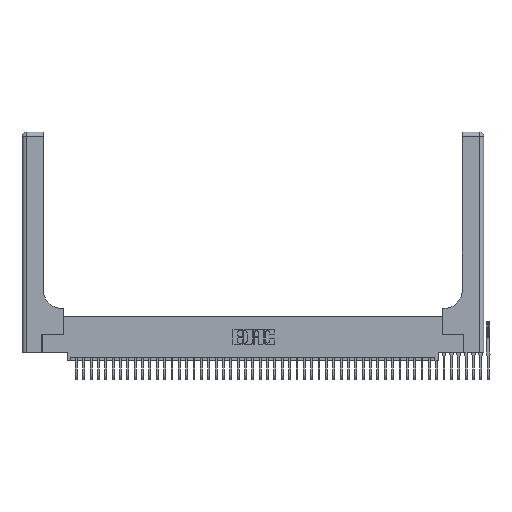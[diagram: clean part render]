
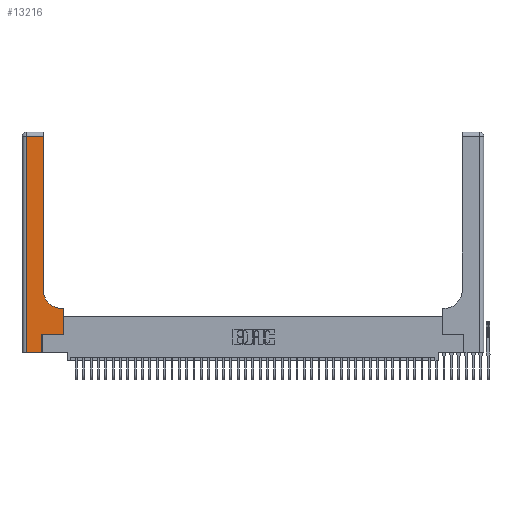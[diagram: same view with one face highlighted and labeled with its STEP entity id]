
A CAD part, top view. The second image highlights one B-rep face of the part: STEP entity #13216.
In plain terms, the highlighted planar face has unit normal (0, 0, 1).
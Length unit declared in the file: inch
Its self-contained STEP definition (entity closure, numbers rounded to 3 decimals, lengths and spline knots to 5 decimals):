
#249 = VECTOR ( 'NONE', #3929, 39.37008 ) ;
#1131 = LINE ( 'NONE', #40847, #33345 ) ;
#1214 = EDGE_CURVE ( 'NONE', #23327, #37470, #10879, .T. ) ;
#1344 = EDGE_CURVE ( 'NONE', #18120, #19431, #21872, .T. ) ;
#1423 = DIRECTION ( 'NONE',  ( -1., 0., 0. ) ) ;
#1444 = VERTEX_POINT ( 'NONE', #2225 ) ;
#2225 = CARTESIAN_POINT ( 'NONE',  ( 0.2915, 2.94, 0.37 ) ) ;
#2936 = LINE ( 'NONE', #36733, #35047 ) ;
#3026 = CARTESIAN_POINT ( 'NONE',  ( 0., 2.94, 0.37 ) ) ;
#3512 = ORIENTED_EDGE ( 'NONE', *, *, #27637, .T. ) ;
#3929 = DIRECTION ( 'NONE',  ( 0., 1., 0. ) ) ;
#4233 = CARTESIAN_POINT ( 'NONE',  ( 0.5415, 0.6, 0.37 ) ) ;
#4406 = DIRECTION ( 'NONE',  ( 0., 0., -1. ) ) ;
#5107 = DIRECTION ( 'NONE',  ( 1., 0., 0. ) ) ;
#5789 = ORIENTED_EDGE ( 'NONE', *, *, #1214, .T. ) ;
#6379 = EDGE_CURVE ( 'NONE', #37470, #1444, #25581, .T. ) ;
#8117 = DIRECTION ( 'NONE',  ( -1., 0., 0. ) ) ;
#8252 = CARTESIAN_POINT ( 'NONE',  ( 0.269, 0.25, 0.37 ) ) ;
#8595 = ORIENTED_EDGE ( 'NONE', *, *, #38573, .T. ) ;
#8697 = EDGE_CURVE ( 'NONE', #21396, #18120, #1131, .T. ) ;
#9582 = DIRECTION ( 'NONE',  ( -1., 0., 0. ) ) ;
#10017 = EDGE_CURVE ( 'NONE', #1444, #25711, #21211, .T. ) ;
#10879 = CIRCLE ( 'NONE', #30761, 0.25 ) ;
#11044 = LINE ( 'NONE', #13742, #19515 ) ;
#12001 = CARTESIAN_POINT ( 'NONE',  ( 0.269, 0.25, 0.37 ) ) ;
#12056 = ORIENTED_EDGE ( 'NONE', *, *, #1344, .T. ) ;
#12397 = LINE ( 'NONE', #12884, #36832 ) ;
#12884 = CARTESIAN_POINT ( 'NONE',  ( 0.06, 3., 0.37 ) ) ;
#13216 = ADVANCED_FACE ( 'NONE', ( #31415 ), #33473, .F. ) ;
#13364 = VECTOR ( 'NONE', #5107, 39.37008 ) ;
#13742 = CARTESIAN_POINT ( 'NONE',  ( 0., 0., 0.37 ) ) ;
#15809 = ORIENTED_EDGE ( 'NONE', *, *, #8697, .T. ) ;
#16067 = DIRECTION ( 'NONE',  ( 0., -1., 0. ) ) ;
#16299 = ORIENTED_EDGE ( 'NONE', *, *, #17195, .T. ) ;
#16336 = ORIENTED_EDGE ( 'NONE', *, *, #6379, .T. ) ;
#17032 = VECTOR ( 'NONE', #41303, 39.37008 ) ;
#17195 = EDGE_CURVE ( 'NONE', #25711, #30571, #12397, .T. ) ;
#17510 = CARTESIAN_POINT ( 'NONE',  ( 0.06, 0., 0.37 ) ) ;
#18120 = VERTEX_POINT ( 'NONE', #12001 ) ;
#18435 = CARTESIAN_POINT ( 'NONE',  ( 0.269, 0., 0.37 ) ) ;
#19431 = VERTEX_POINT ( 'NONE', #31596 ) ;
#19515 = VECTOR ( 'NONE', #32883, 39.37008 ) ;
#19549 = EDGE_LOOP ( 'NONE', ( #16336, #27543, #16299, #30661, #15809, #12056, #8595, #3512, #5789 ) ) ;
#19664 = AXIS2_PLACEMENT_3D ( 'NONE', #39839, #20764, #1423 ) ;
#20764 = DIRECTION ( 'NONE',  ( 0., 0., -1. ) ) ;
#21211 = LINE ( 'NONE', #3026, #37180 ) ;
#21396 = VERTEX_POINT ( 'NONE', #18435 ) ;
#21872 = LINE ( 'NONE', #8252, #13364 ) ;
#23327 = VERTEX_POINT ( 'NONE', #4233 ) ;
#23649 = CARTESIAN_POINT ( 'NONE',  ( 0.5415, 0.85, 0.37 ) ) ;
#24467 = CARTESIAN_POINT ( 'NONE',  ( 0.5585, 0.6, 0.37 ) ) ;
#25465 = CARTESIAN_POINT ( 'NONE',  ( 0.2915, 3., 0.37 ) ) ;
#25581 = LINE ( 'NONE', #25465, #17032 ) ;
#25711 = VERTEX_POINT ( 'NONE', #36655 ) ;
#26023 = LINE ( 'NONE', #29587, #249 ) ;
#26857 = DIRECTION ( 'NONE',  ( 1., 0., 0. ) ) ;
#27543 = ORIENTED_EDGE ( 'NONE', *, *, #10017, .T. ) ;
#27637 = EDGE_CURVE ( 'NONE', #38161, #23327, #2936, .T. ) ;
#29587 = CARTESIAN_POINT ( 'NONE',  ( 0.5585, 0.25, 0.37 ) ) ;
#30571 = VERTEX_POINT ( 'NONE', #17510 ) ;
#30661 = ORIENTED_EDGE ( 'NONE', *, *, #32097, .T. ) ;
#30761 = AXIS2_PLACEMENT_3D ( 'NONE', #23649, #4406, #26857 ) ;
#31415 = FACE_OUTER_BOUND ( 'NONE', #19549, .T. ) ;
#31596 = CARTESIAN_POINT ( 'NONE',  ( 0.5585, 0.25, 0.37 ) ) ;
#32097 = EDGE_CURVE ( 'NONE', #30571, #21396, #11044, .T. ) ;
#32883 = DIRECTION ( 'NONE',  ( 1., 0., 0. ) ) ;
#33345 = VECTOR ( 'NONE', #34631, 39.37008 ) ;
#33473 = PLANE ( 'NONE',  #19664 ) ;
#33581 = CARTESIAN_POINT ( 'NONE',  ( 0.2915, 0.85, 0.37 ) ) ;
#34631 = DIRECTION ( 'NONE',  ( 0., 1., 0. ) ) ;
#35047 = VECTOR ( 'NONE', #8117, 39.37008 ) ;
#36655 = CARTESIAN_POINT ( 'NONE',  ( 0.06, 2.94, 0.37 ) ) ;
#36733 = CARTESIAN_POINT ( 'NONE',  ( 0.2915, 0.6, 0.37 ) ) ;
#36832 = VECTOR ( 'NONE', #16067, 39.37008 ) ;
#37180 = VECTOR ( 'NONE', #9582, 39.37008 ) ;
#37470 = VERTEX_POINT ( 'NONE', #33581 ) ;
#38161 = VERTEX_POINT ( 'NONE', #24467 ) ;
#38573 = EDGE_CURVE ( 'NONE', #19431, #38161, #26023, .T. ) ;
#39839 = CARTESIAN_POINT ( 'NONE',  ( 0., 3., 0.37 ) ) ;
#40847 = CARTESIAN_POINT ( 'NONE',  ( 0.269, 0., 0.37 ) ) ;
#41303 = DIRECTION ( 'NONE',  ( 0., 1., 0. ) ) ;
